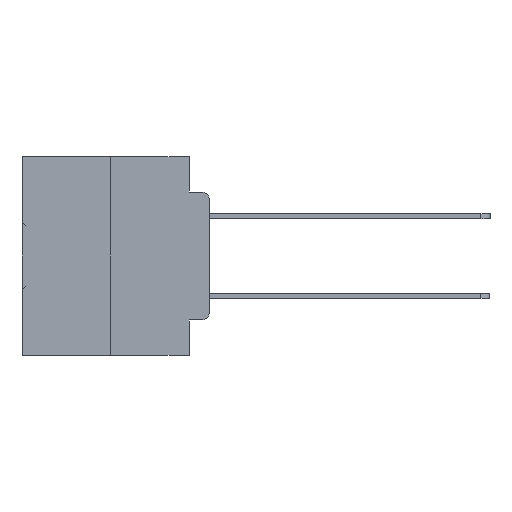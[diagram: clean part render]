
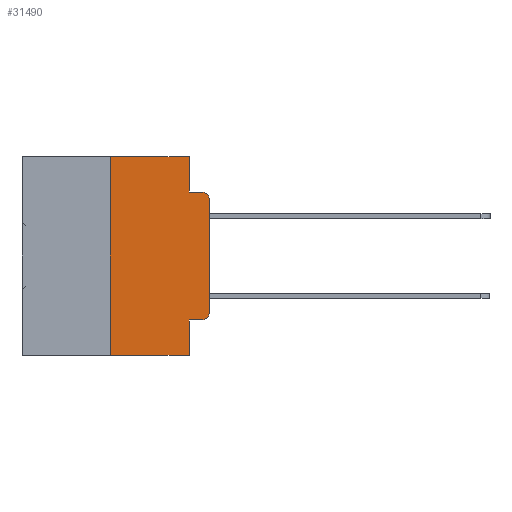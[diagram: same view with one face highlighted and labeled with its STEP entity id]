
A CAD part, left-side view. The second image highlights one B-rep face of the part: STEP entity #31490.
In plain terms, the highlighted planar face has unit normal (-1, 0, 0).
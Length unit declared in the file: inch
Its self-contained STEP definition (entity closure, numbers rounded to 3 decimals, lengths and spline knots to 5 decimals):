
#401 = VERTEX_POINT ( 'NONE', #22742 ) ;
#604 = PLANE ( 'NONE',  #19893 ) ;
#660 = VERTEX_POINT ( 'NONE', #9714 ) ;
#1096 = LINE ( 'NONE', #7139, #28824 ) ;
#1922 = AXIS2_PLACEMENT_3D ( 'NONE', #4487, #23354, #7261 ) ;
#1923 = VECTOR ( 'NONE', #15630, 39.37008 ) ;
#2617 = VERTEX_POINT ( 'NONE', #33747 ) ;
#3328 = ORIENTED_EDGE ( 'NONE', *, *, #7174, .T. ) ;
#3375 = DIRECTION ( 'NONE',  ( 1., 0., 0. ) ) ;
#3437 = CARTESIAN_POINT ( 'NONE',  ( 0., 0.051, 0. ) ) ;
#4487 = CARTESIAN_POINT ( 'NONE',  ( 0., 0.02, -0.1085 ) ) ;
#4502 = ORIENTED_EDGE ( 'NONE', *, *, #5351, .T. ) ;
#5351 = EDGE_CURVE ( 'NONE', #660, #401, #17930, .T. ) ;
#5503 = ORIENTED_EDGE ( 'NONE', *, *, #21897, .T. ) ;
#5817 = VERTEX_POINT ( 'NONE', #20745 ) ;
#6087 = VECTOR ( 'NONE', #23764, 39.37008 ) ;
#6221 = ORIENTED_EDGE ( 'NONE', *, *, #30426, .T. ) ;
#6810 = DIRECTION ( 'NONE',  ( 0., 0., -1. ) ) ;
#7139 = CARTESIAN_POINT ( 'NONE',  ( 0., 0.051, -0.4115 ) ) ;
#7174 = EDGE_CURVE ( 'NONE', #25296, #2617, #29589, .T. ) ;
#7261 = DIRECTION ( 'NONE',  ( 0., 0., -1. ) ) ;
#7291 = LINE ( 'NONE', #32120, #14530 ) ;
#7616 = CARTESIAN_POINT ( 'NONE',  ( 0., 0.051, -0.0885 ) ) ;
#7748 = CIRCLE ( 'NONE', #17450, 0.02 ) ;
#7807 = VECTOR ( 'NONE', #30047, 39.37008 ) ;
#7954 = ORIENTED_EDGE ( 'NONE', *, *, #9479, .F. ) ;
#8190 = VERTEX_POINT ( 'NONE', #26949 ) ;
#9479 = EDGE_CURVE ( 'NONE', #12170, #22312, #29891, .T. ) ;
#9714 = CARTESIAN_POINT ( 'NONE',  ( 0., 0., -0.3915 ) ) ;
#10641 = EDGE_CURVE ( 'NONE', #25296, #22359, #7291, .T. ) ;
#12170 = VERTEX_POINT ( 'NONE', #7616 ) ;
#12301 = ORIENTED_EDGE ( 'NONE', *, *, #15418, .F. ) ;
#12466 = LINE ( 'NONE', #18463, #6087 ) ;
#12886 = CARTESIAN_POINT ( 'NONE',  ( 0., 0.473, -0.5 ) ) ;
#13072 = CARTESIAN_POINT ( 'NONE',  ( 0., 0.25, -0.5 ) ) ;
#13965 = CARTESIAN_POINT ( 'NONE',  ( 0., 0.051, 0. ) ) ;
#14021 = ORIENTED_EDGE ( 'NONE', *, *, #27830, .T. ) ;
#14530 = VECTOR ( 'NONE', #16398, 39.37008 ) ;
#15418 = EDGE_CURVE ( 'NONE', #5817, #2617, #32074, .T. ) ;
#15630 = DIRECTION ( 'NONE',  ( 0., -1., 0. ) ) ;
#16320 = DIRECTION ( 'NONE',  ( -1., 0., 0. ) ) ;
#16355 = CARTESIAN_POINT ( 'NONE',  ( 0., 0., 0. ) ) ;
#16398 = DIRECTION ( 'NONE',  ( 0., 0., 1. ) ) ;
#16472 = ORIENTED_EDGE ( 'NONE', *, *, #18553, .F. ) ;
#17450 = AXIS2_PLACEMENT_3D ( 'NONE', #32038, #16320, #6810 ) ;
#17930 = LINE ( 'NONE', #16355, #24118 ) ;
#18054 = CARTESIAN_POINT ( 'NONE',  ( 0., 0.25, 0. ) ) ;
#18150 = VECTOR ( 'NONE', #19368, 39.37008 ) ;
#18463 = CARTESIAN_POINT ( 'NONE',  ( 0., 0.473, 0. ) ) ;
#18553 = EDGE_CURVE ( 'NONE', #8190, #12170, #19001, .T. ) ;
#19001 = LINE ( 'NONE', #3437, #25177 ) ;
#19368 = DIRECTION ( 'NONE',  ( 0., 0., -1. ) ) ;
#19893 = AXIS2_PLACEMENT_3D ( 'NONE', #24773, #3375, #22239 ) ;
#20745 = CARTESIAN_POINT ( 'NONE',  ( 0., 0.051, -0.4115 ) ) ;
#21165 = EDGE_CURVE ( 'NONE', #22359, #8190, #12466, .T. ) ;
#21897 = EDGE_CURVE ( 'NONE', #26382, #660, #7748, .T. ) ;
#22239 = DIRECTION ( 'NONE',  ( 0., 0., -1. ) ) ;
#22312 = VERTEX_POINT ( 'NONE', #23257 ) ;
#22359 = VERTEX_POINT ( 'NONE', #18054 ) ;
#22742 = CARTESIAN_POINT ( 'NONE',  ( 0., 0., -0.1085 ) ) ;
#23257 = CARTESIAN_POINT ( 'NONE',  ( 0., 0.02, -0.0885 ) ) ;
#23354 = DIRECTION ( 'NONE',  ( -1., 0., 0. ) ) ;
#23764 = DIRECTION ( 'NONE',  ( 0., -1., 0. ) ) ;
#23936 = ORIENTED_EDGE ( 'NONE', *, *, #21165, .F. ) ;
#24118 = VECTOR ( 'NONE', #24218, 39.37008 ) ;
#24218 = DIRECTION ( 'NONE',  ( 0., 0., 1. ) ) ;
#24773 = CARTESIAN_POINT ( 'NONE',  ( 0., 0.473, 0. ) ) ;
#25058 = CARTESIAN_POINT ( 'NONE',  ( 0., 0.02, -0.4115 ) ) ;
#25177 = VECTOR ( 'NONE', #27712, 39.37008 ) ;
#25296 = VERTEX_POINT ( 'NONE', #13072 ) ;
#25878 = DIRECTION ( 'NONE',  ( 0., -1., 0. ) ) ;
#26326 = CIRCLE ( 'NONE', #1922, 0.02 ) ;
#26382 = VERTEX_POINT ( 'NONE', #25058 ) ;
#26845 = ORIENTED_EDGE ( 'NONE', *, *, #10641, .F. ) ;
#26864 = CARTESIAN_POINT ( 'NONE',  ( 0., 0.051, -0.0885 ) ) ;
#26949 = CARTESIAN_POINT ( 'NONE',  ( 0., 0.051, 0. ) ) ;
#27712 = DIRECTION ( 'NONE',  ( 0., 0., -1. ) ) ;
#27830 = EDGE_CURVE ( 'NONE', #5817, #26382, #1096, .T. ) ;
#28824 = VECTOR ( 'NONE', #25878, 39.37008 ) ;
#29589 = LINE ( 'NONE', #12886, #1923 ) ;
#29676 = EDGE_LOOP ( 'NONE', ( #4502, #6221, #7954, #16472, #23936, #26845, #3328, #12301, #14021, #5503 ) ) ;
#29891 = LINE ( 'NONE', #26864, #7807 ) ;
#30047 = DIRECTION ( 'NONE',  ( 0., -1., 0. ) ) ;
#30426 = EDGE_CURVE ( 'NONE', #401, #22312, #26326, .T. ) ;
#31490 = ADVANCED_FACE ( 'NONE', ( #33583 ), #604, .F. ) ;
#32038 = CARTESIAN_POINT ( 'NONE',  ( 0., 0.02, -0.3915 ) ) ;
#32074 = LINE ( 'NONE', #13965, #18150 ) ;
#32120 = CARTESIAN_POINT ( 'NONE',  ( 0., 0.25, 0. ) ) ;
#33583 = FACE_OUTER_BOUND ( 'NONE', #29676, .T. ) ;
#33747 = CARTESIAN_POINT ( 'NONE',  ( 0., 0.051, -0.5 ) ) ;
